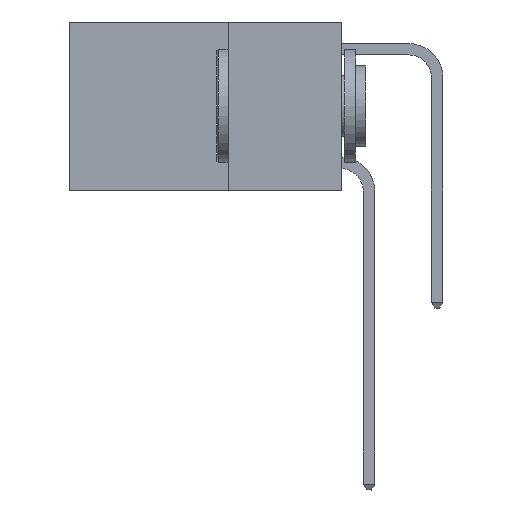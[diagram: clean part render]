
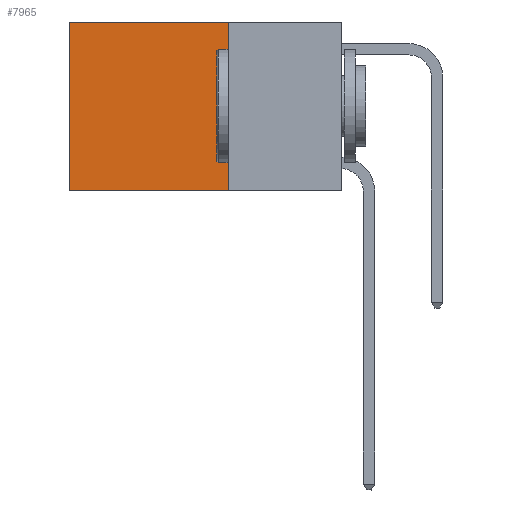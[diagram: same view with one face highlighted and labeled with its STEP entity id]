
A CAD part, left-side view. The second image highlights one B-rep face of the part: STEP entity #7965.
In plain terms, the highlighted planar face has unit normal (-1, 0, 0).
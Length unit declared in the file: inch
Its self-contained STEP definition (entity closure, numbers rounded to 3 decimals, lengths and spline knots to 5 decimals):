
#237 = DIRECTION ( 'NONE',  ( 0., 1., 0. ) ) ;
#599 = LINE ( 'NONE', #16027, #10797 ) ;
#997 = DIRECTION ( 'NONE',  ( 0., 1., 0. ) ) ;
#1020 = CARTESIAN_POINT ( 'NONE',  ( 0.2625, 0.25, 0. ) ) ;
#1463 = EDGE_CURVE ( 'NONE', #5442, #13272, #599, .T. ) ;
#2476 = DIRECTION ( 'NONE',  ( 0., 0., -1. ) ) ;
#3581 = CARTESIAN_POINT ( 'NONE',  ( 0.2625, 0.6, 0. ) ) ;
#3692 = CARTESIAN_POINT ( 'NONE',  ( 0.2625, 0.6, 0. ) ) ;
#3808 = DIRECTION ( 'NONE',  ( 0., 0., -1. ) ) ;
#4234 = LINE ( 'NONE', #10126, #14662 ) ;
#4559 = EDGE_CURVE ( 'NONE', #10378, #15404, #4234, .T. ) ;
#5293 = EDGE_CURVE ( 'NONE', #10378, #5442, #11378, .T. ) ;
#5442 = VERTEX_POINT ( 'NONE', #12129 ) ;
#5860 = FACE_OUTER_BOUND ( 'NONE', #7654, .T. ) ;
#6068 = ORIENTED_EDGE ( 'NONE', *, *, #4559, .T. ) ;
#6149 = ORIENTED_EDGE ( 'NONE', *, *, #5293, .F. ) ;
#7013 = VECTOR ( 'NONE', #3808, 39.37008 ) ;
#7586 = CARTESIAN_POINT ( 'NONE',  ( 0.2625, 0.25, 0. ) ) ;
#7654 = EDGE_LOOP ( 'NONE', ( #15670, #17613, #6149, #6068 ) ) ;
#7753 = CARTESIAN_POINT ( 'NONE',  ( 0.2625, 0.6, -0.37 ) ) ;
#7965 = ADVANCED_FACE ( 'NONE', ( #5860 ), #13497, .F. ) ;
#10126 = CARTESIAN_POINT ( 'NONE',  ( 0.2625, 0.25, 0. ) ) ;
#10378 = VERTEX_POINT ( 'NONE', #11337 ) ;
#10764 = DIRECTION ( 'NONE',  ( 1., 0., 0. ) ) ;
#10797 = VECTOR ( 'NONE', #997, 39.37008 ) ;
#11337 = CARTESIAN_POINT ( 'NONE',  ( 0.2625, 0.25, 0. ) ) ;
#11378 = LINE ( 'NONE', #7586, #17879 ) ;
#12129 = CARTESIAN_POINT ( 'NONE',  ( 0.2625, 0.25, -0.37 ) ) ;
#12171 = AXIS2_PLACEMENT_3D ( 'NONE', #1020, #10764, #2476 ) ;
#13002 = DIRECTION ( 'NONE',  ( 0., 0., -1. ) ) ;
#13272 = VERTEX_POINT ( 'NONE', #7753 ) ;
#13497 = PLANE ( 'NONE',  #12171 ) ;
#14603 = LINE ( 'NONE', #3692, #7013 ) ;
#14662 = VECTOR ( 'NONE', #237, 39.37008 ) ;
#15404 = VERTEX_POINT ( 'NONE', #3581 ) ;
#15670 = ORIENTED_EDGE ( 'NONE', *, *, #16366, .T. ) ;
#16027 = CARTESIAN_POINT ( 'NONE',  ( 0.2625, 0.25, -0.37 ) ) ;
#16366 = EDGE_CURVE ( 'NONE', #15404, #13272, #14603, .T. ) ;
#17613 = ORIENTED_EDGE ( 'NONE', *, *, #1463, .F. ) ;
#17879 = VECTOR ( 'NONE', #13002, 39.37008 ) ;
